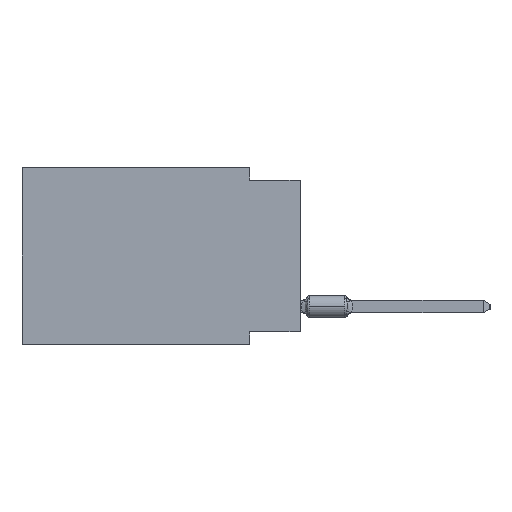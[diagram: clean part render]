
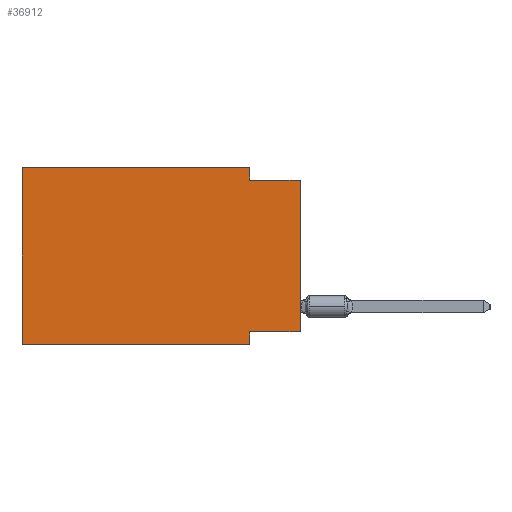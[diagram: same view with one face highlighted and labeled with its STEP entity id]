
A CAD part, left-side view. The second image highlights one B-rep face of the part: STEP entity #36912.
In plain terms, the highlighted planar face has unit normal (-1, 0, 0).
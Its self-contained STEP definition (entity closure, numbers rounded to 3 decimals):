
#147 = CARTESIAN_POINT ( 'NONE',  ( 0., 13.97, 0. ) ) ;
#265 = CARTESIAN_POINT ( 'NONE',  ( 0., 13.97, -8.89 ) ) ;
#380 = CARTESIAN_POINT ( 'NONE',  ( 0., 2.54, 0. ) ) ;
#2736 = ORIENTED_EDGE ( 'NONE', *, *, #14527, .F. ) ;
#3444 = CARTESIAN_POINT ( 'NONE',  ( 0., 2.54, -8.89 ) ) ;
#4800 = DIRECTION ( 'NONE',  ( 0., 0., -1. ) ) ;
#4867 = VECTOR ( 'NONE', #58748, 1000. ) ;
#6049 = DIRECTION ( 'NONE',  ( 1., 0., 0. ) ) ;
#9746 = VECTOR ( 'NONE', #48444, 1000. ) ;
#10192 = CARTESIAN_POINT ( 'NONE',  ( 0., 13.97, 0. ) ) ;
#12654 = VERTEX_POINT ( 'NONE', #23006 ) ;
#14502 = CARTESIAN_POINT ( 'NONE',  ( 0., 0., -0.635 ) ) ;
#14527 = EDGE_CURVE ( 'NONE', #12654, #30699, #34070, .T. ) ;
#14560 = CARTESIAN_POINT ( 'NONE',  ( 0., 0., -8.255 ) ) ;
#15292 = LINE ( 'NONE', #48250, #32658 ) ;
#16545 = LINE ( 'NONE', #48802, #9746 ) ;
#17742 = VERTEX_POINT ( 'NONE', #380 ) ;
#21355 = VECTOR ( 'NONE', #4800, 1000. ) ;
#21383 = DIRECTION ( 'NONE',  ( 0., 1., 0. ) ) ;
#22102 = DIRECTION ( 'NONE',  ( 0., -1., 0. ) ) ;
#23006 = CARTESIAN_POINT ( 'NONE',  ( 0., 2.54, -8.255 ) ) ;
#24388 = EDGE_CURVE ( 'NONE', #27250, #40577, #30823, .T. ) ;
#24938 = EDGE_CURVE ( 'NONE', #43729, #12654, #48966, .T. ) ;
#25404 = VERTEX_POINT ( 'NONE', #10192 ) ;
#27250 = VERTEX_POINT ( 'NONE', #47333 ) ;
#27721 = LINE ( 'NONE', #147, #38101 ) ;
#29381 = CARTESIAN_POINT ( 'NONE',  ( 0., 13.97, -8.89 ) ) ;
#30699 = VERTEX_POINT ( 'NONE', #3444 ) ;
#30823 = LINE ( 'NONE', #37263, #4867 ) ;
#31367 = ORIENTED_EDGE ( 'NONE', *, *, #53942, .F. ) ;
#32215 = DIRECTION ( 'NONE',  ( 0., 0., -1. ) ) ;
#32658 = VECTOR ( 'NONE', #42183, 1000. ) ;
#33104 = ORIENTED_EDGE ( 'NONE', *, *, #51621, .F. ) ;
#34070 = LINE ( 'NONE', #67020, #21355 ) ;
#36912 = ADVANCED_FACE ( 'NONE', ( #37954 ), #43325, .F. ) ;
#37263 = CARTESIAN_POINT ( 'NONE',  ( 0., 0., -0.635 ) ) ;
#37954 = FACE_OUTER_BOUND ( 'NONE', #65373, .T. ) ;
#38101 = VECTOR ( 'NONE', #49573, 1000. ) ;
#40577 = VERTEX_POINT ( 'NONE', #14502 ) ;
#41437 = EDGE_CURVE ( 'NONE', #43729, #40577, #15292, .T. ) ;
#42183 = DIRECTION ( 'NONE',  ( 0., 0., 1. ) ) ;
#42470 = LINE ( 'NONE', #42819, #63418 ) ;
#42819 = CARTESIAN_POINT ( 'NONE',  ( 0., 13.97, 0. ) ) ;
#43325 = PLANE ( 'NONE',  #53726 ) ;
#43729 = VERTEX_POINT ( 'NONE', #14560 ) ;
#44437 = ORIENTED_EDGE ( 'NONE', *, *, #41437, .T. ) ;
#45959 = VERTEX_POINT ( 'NONE', #29381 ) ;
#47333 = CARTESIAN_POINT ( 'NONE',  ( 0., 2.54, -0.635 ) ) ;
#48250 = CARTESIAN_POINT ( 'NONE',  ( 0., 0., 0. ) ) ;
#48444 = DIRECTION ( 'NONE',  ( 0., 0., -1. ) ) ;
#48802 = CARTESIAN_POINT ( 'NONE',  ( 0., 2.54, 0. ) ) ;
#48966 = LINE ( 'NONE', #54676, #57556 ) ;
#49573 = DIRECTION ( 'NONE',  ( 0., -1., 0. ) ) ;
#49694 = LINE ( 'NONE', #265, #70491 ) ;
#51621 = EDGE_CURVE ( 'NONE', #45959, #25404, #42470, .T. ) ;
#51737 = ORIENTED_EDGE ( 'NONE', *, *, #24388, .F. ) ;
#53726 = AXIS2_PLACEMENT_3D ( 'NONE', #59794, #6049, #32215 ) ;
#53942 = EDGE_CURVE ( 'NONE', #17742, #27250, #16545, .T. ) ;
#54676 = CARTESIAN_POINT ( 'NONE',  ( 0., 0., -8.255 ) ) ;
#56560 = EDGE_CURVE ( 'NONE', #45959, #30699, #49694, .T. ) ;
#56626 = ORIENTED_EDGE ( 'NONE', *, *, #56560, .T. ) ;
#57556 = VECTOR ( 'NONE', #21383, 1000. ) ;
#58748 = DIRECTION ( 'NONE',  ( 0., -1., 0. ) ) ;
#59794 = CARTESIAN_POINT ( 'NONE',  ( 0., 13.97, 0. ) ) ;
#62668 = ORIENTED_EDGE ( 'NONE', *, *, #66416, .F. ) ;
#63418 = VECTOR ( 'NONE', #70398, 1000. ) ;
#64274 = ORIENTED_EDGE ( 'NONE', *, *, #24938, .F. ) ;
#65373 = EDGE_LOOP ( 'NONE', ( #44437, #51737, #31367, #62668, #33104, #56626, #2736, #64274 ) ) ;
#66416 = EDGE_CURVE ( 'NONE', #25404, #17742, #27721, .T. ) ;
#67020 = CARTESIAN_POINT ( 'NONE',  ( 0., 2.54, -8.89 ) ) ;
#70398 = DIRECTION ( 'NONE',  ( 0., 0., 1. ) ) ;
#70491 = VECTOR ( 'NONE', #22102, 1000. ) ;
